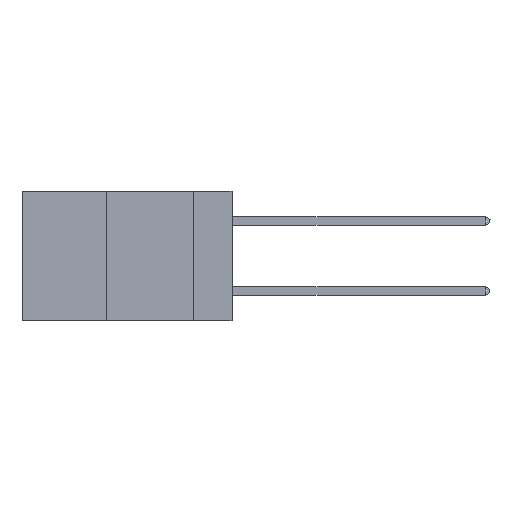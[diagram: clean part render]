
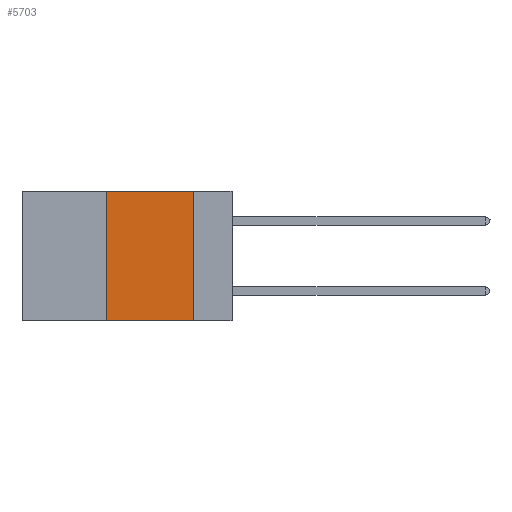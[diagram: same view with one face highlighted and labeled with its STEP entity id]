
A CAD part, left-side view. The second image highlights one B-rep face of the part: STEP entity #5703.
In plain terms, the highlighted planar face has unit normal (-1, 0, 0).
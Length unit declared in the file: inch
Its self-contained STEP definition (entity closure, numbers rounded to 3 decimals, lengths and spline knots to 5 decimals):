
#17 = VECTOR ( 'NONE', #2624, 39.37008 ) ;
#562 = EDGE_CURVE ( 'NONE', #20239, #2741, #15986, .T. ) ;
#903 = VECTOR ( 'NONE', #11975, 39.37008 ) ;
#1727 = EDGE_CURVE ( 'NONE', #2237, #20239, #23939, .T. ) ;
#2237 = VERTEX_POINT ( 'NONE', #22186 ) ;
#2624 = DIRECTION ( 'NONE',  ( 0., 0., -1. ) ) ;
#2741 = VERTEX_POINT ( 'NONE', #18647 ) ;
#2803 = CARTESIAN_POINT ( 'NONE',  ( 0., 0.6, -0.37 ) ) ;
#3470 = CARTESIAN_POINT ( 'NONE',  ( 0., 0.36, -0.37 ) ) ;
#3979 = LINE ( 'NONE', #9788, #16403 ) ;
#4013 = VECTOR ( 'NONE', #12697, 39.37008 ) ;
#4352 = CARTESIAN_POINT ( 'NONE',  ( 0., 0.11, 0. ) ) ;
#5353 = DIRECTION ( 'NONE',  ( 0., 0., -1. ) ) ;
#5703 = ADVANCED_FACE ( 'NONE', ( #6964 ), #8822, .F. ) ;
#6964 = FACE_OUTER_BOUND ( 'NONE', #14535, .T. ) ;
#8822 = PLANE ( 'NONE',  #11752 ) ;
#9788 = CARTESIAN_POINT ( 'NONE',  ( 0., 0.36, 0. ) ) ;
#10314 = ORIENTED_EDGE ( 'NONE', *, *, #13888, .T. ) ;
#10985 = CARTESIAN_POINT ( 'NONE',  ( 0., 0.11, 0. ) ) ;
#11143 = ORIENTED_EDGE ( 'NONE', *, *, #562, .F. ) ;
#11752 = AXIS2_PLACEMENT_3D ( 'NONE', #16359, #12537, #5353 ) ;
#11975 = DIRECTION ( 'NONE',  ( 0., -1., 0. ) ) ;
#12537 = DIRECTION ( 'NONE',  ( 1., 0., 0. ) ) ;
#12697 = DIRECTION ( 'NONE',  ( 0., -1., 0. ) ) ;
#13217 = ORIENTED_EDGE ( 'NONE', *, *, #16440, .F. ) ;
#13888 = EDGE_CURVE ( 'NONE', #18427, #2741, #19728, .T. ) ;
#14535 = EDGE_LOOP ( 'NONE', ( #11143, #15620, #13217, #10314 ) ) ;
#15125 = DIRECTION ( 'NONE',  ( 0., 0., 1. ) ) ;
#15620 = ORIENTED_EDGE ( 'NONE', *, *, #1727, .F. ) ;
#15986 = LINE ( 'NONE', #4352, #17 ) ;
#16359 = CARTESIAN_POINT ( 'NONE',  ( 0., 0.6, 0. ) ) ;
#16403 = VECTOR ( 'NONE', #15125, 39.37008 ) ;
#16440 = EDGE_CURVE ( 'NONE', #18427, #2237, #3979, .T. ) ;
#18427 = VERTEX_POINT ( 'NONE', #3470 ) ;
#18647 = CARTESIAN_POINT ( 'NONE',  ( 0., 0.11, -0.37 ) ) ;
#19728 = LINE ( 'NONE', #2803, #903 ) ;
#20239 = VERTEX_POINT ( 'NONE', #10985 ) ;
#22096 = CARTESIAN_POINT ( 'NONE',  ( 0., 0.6, 0. ) ) ;
#22186 = CARTESIAN_POINT ( 'NONE',  ( 0., 0.36, 0. ) ) ;
#23939 = LINE ( 'NONE', #22096, #4013 ) ;
